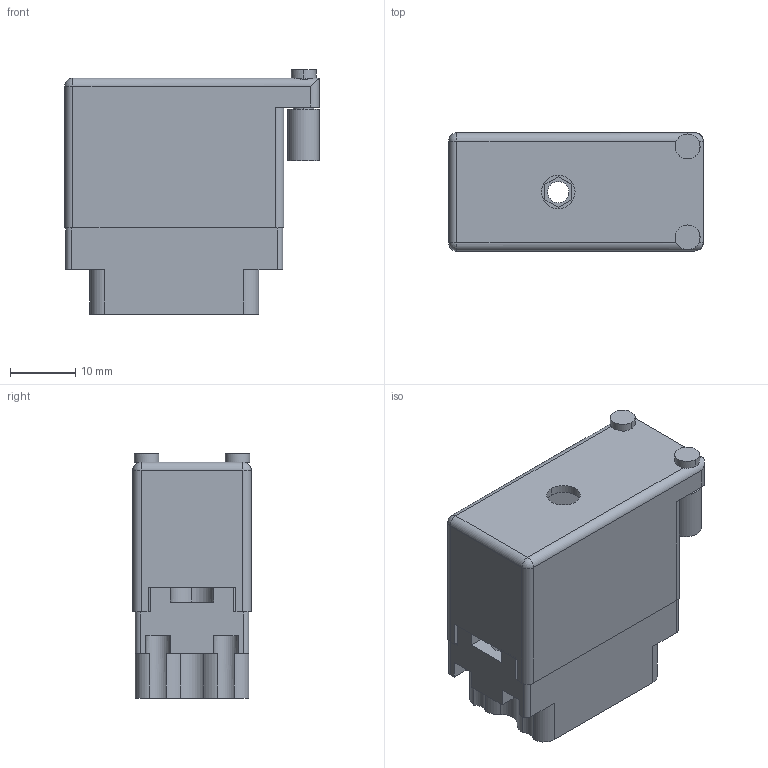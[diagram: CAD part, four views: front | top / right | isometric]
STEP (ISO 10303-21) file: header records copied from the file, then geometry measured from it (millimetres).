
FILE_DESCRIPTION (( 'STEP AP203' ), '1' );
FILE_NAME ('519-014-501-350.STEP', '2020-09-09T15:27:43', ( '' ), ( '' ), 'SwSTEP 2.0', 'SolidWorks 2020', '' );
FILE_SCHEMA (( 'CONFIG_CONTROL_DESIGN' ));
Length unit declared in the file: inch
Products named in the file (4): 516-292-001_501 Contact; 516-230-001_Metal - 020 Side Entry; 519-014-501-350; 519 Plug Insulator_014
Assembly tree (16 placements, depth 2):
  519-014-501-350
    519 Plug Insulator_014
    516-292-001_501 Contact  x14
    516-230-001_Metal - 020 Side Entry
Bounding box: 39.12 x 18.16 x 37.52 mm (x, y, z)
Volume: 9367.4 mm3; surface area: 14547.7 mm2
Topology: 16 solids, 16 shells, 1568 faces, 4535 edges, 3006 vertices
Faces by surface type: plane 938, cylinder 542, bspline 84, cone 2, sphere 2
Entity records: 21966 total; most frequent: CARTESIAN_POINT 4014, ORIENTED_EDGE 3658, DIRECTION 3575, EDGE_CURVE 1829, LINE 1295, VECTOR 1295, VERTEX_POINT 1212, AXIS2_PLACEMENT_3D 1140
